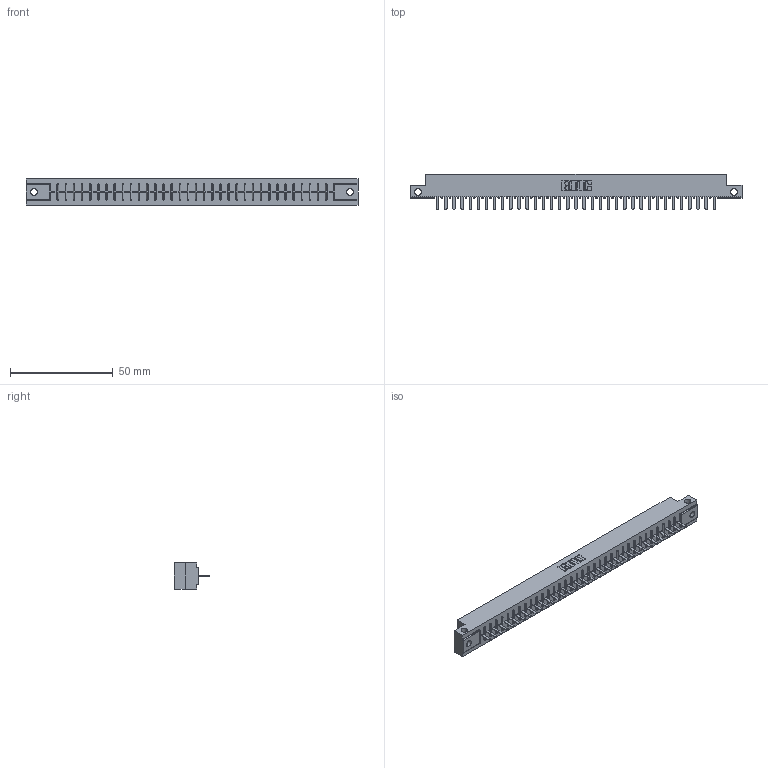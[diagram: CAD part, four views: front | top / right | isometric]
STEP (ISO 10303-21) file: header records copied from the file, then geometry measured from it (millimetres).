
FILE_DESCRIPTION (( 'STEP AP203' ), '1' );
FILE_NAME ('316-035-520-112.STEP', '2020-09-20T21:24:25', ( '' ), ( '' ), 'SwSTEP 2.0', 'SolidWorks 2020', '' );
FILE_SCHEMA (( 'CONFIG_CONTROL_DESIGN' ));
Length unit declared in the file: inch
Products named in the file (3): 316-035-520-112; 306 Part_.128 Dia; 306-290-001_120
Assembly tree (36 placements, depth 2):
  316-035-520-112
    306 Part_.128 Dia
    306-290-001_120  x35
Bounding box: 161.7 x 17.12 x 12.7 mm (x, y, z)
Volume: 17627.7 mm3; surface area: 18055.4 mm2
Topology: 36 solids, 36 shells, 2578 faces, 7247 edges, 4638 vertices
Faces by surface type: plane 1713, cylinder 725, sphere 140
Entity records: 33908 total; most frequent: CARTESIAN_POINT 5740, ORIENTED_EDGE 5646, DIRECTION 5599, EDGE_CURVE 2823, LINE 2189, VECTOR 2189, VERTEX_POINT 1782, AXIS2_PLACEMENT_3D 1705
